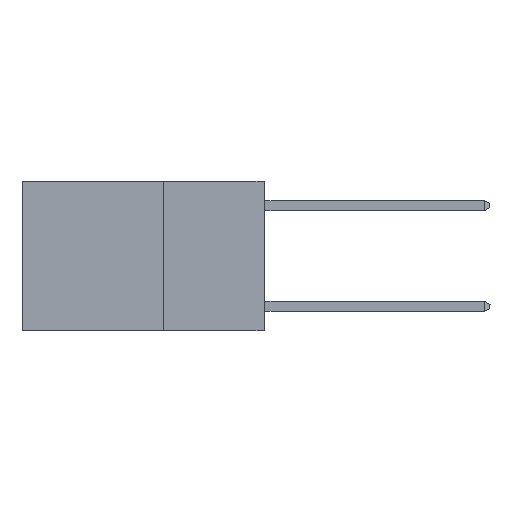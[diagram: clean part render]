
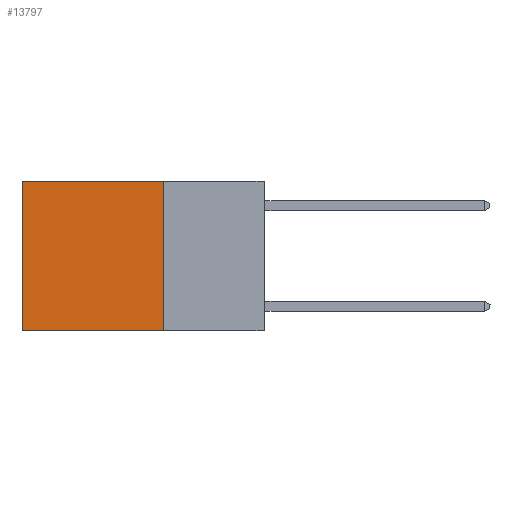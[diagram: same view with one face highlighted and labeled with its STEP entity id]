
A CAD part, left-side view. The second image highlights one B-rep face of the part: STEP entity #13797.
In plain terms, the highlighted planar face has unit normal (-1, 0, 0).
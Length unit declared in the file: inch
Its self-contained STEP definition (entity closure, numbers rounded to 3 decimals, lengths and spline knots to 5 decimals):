
#148 = CARTESIAN_POINT ( 'NONE',  ( 0.2625, 0.25, 0. ) ) ;
#158 = AXIS2_PLACEMENT_3D ( 'NONE', #20457, #4728, #18549 ) ;
#2574 = ORIENTED_EDGE ( 'NONE', *, *, #3627, .T. ) ;
#2757 = PLANE ( 'NONE',  #158 ) ;
#3167 = LINE ( 'NONE', #21795, #13043 ) ;
#3627 = EDGE_CURVE ( 'NONE', #9972, #22703, #16249, .T. ) ;
#4336 = VERTEX_POINT ( 'NONE', #22454 ) ;
#4482 = DIRECTION ( 'NONE',  ( 0., 1., 0. ) ) ;
#4728 = DIRECTION ( 'NONE',  ( 1., 0., 0. ) ) ;
#6208 = EDGE_CURVE ( 'NONE', #4336, #9972, #15558, .T. ) ;
#6687 = DIRECTION ( 'NONE',  ( 0., 0., -1. ) ) ;
#6780 = CARTESIAN_POINT ( 'NONE',  ( 0.2625, 0.6, 0. ) ) ;
#7903 = FACE_OUTER_BOUND ( 'NONE', #21401, .T. ) ;
#8451 = CARTESIAN_POINT ( 'NONE',  ( 0.2625, 0.25, 0. ) ) ;
#8717 = CARTESIAN_POINT ( 'NONE',  ( 0.2625, 0.6, 0. ) ) ;
#9972 = VERTEX_POINT ( 'NONE', #8717 ) ;
#10179 = EDGE_CURVE ( 'NONE', #4336, #18437, #20729, .T. ) ;
#12616 = CARTESIAN_POINT ( 'NONE',  ( 0.2625, 0.6, -0.37 ) ) ;
#13043 = VECTOR ( 'NONE', #17857, 39.37008 ) ;
#13797 = ADVANCED_FACE ( 'NONE', ( #7903 ), #2757, .F. ) ;
#15558 = LINE ( 'NONE', #8451, #20790 ) ;
#16169 = EDGE_CURVE ( 'NONE', #18437, #22703, #3167, .T. ) ;
#16249 = LINE ( 'NONE', #6780, #17508 ) ;
#17508 = VECTOR ( 'NONE', #6687, 39.37008 ) ;
#17857 = DIRECTION ( 'NONE',  ( 0., 1., 0. ) ) ;
#17922 = DIRECTION ( 'NONE',  ( 0., 0., -1. ) ) ;
#18437 = VERTEX_POINT ( 'NONE', #24619 ) ;
#18549 = DIRECTION ( 'NONE',  ( 0., 0., -1. ) ) ;
#20413 = ORIENTED_EDGE ( 'NONE', *, *, #10179, .F. ) ;
#20457 = CARTESIAN_POINT ( 'NONE',  ( 0.2625, 0.25, 0. ) ) ;
#20729 = LINE ( 'NONE', #148, #24608 ) ;
#20790 = VECTOR ( 'NONE', #4482, 39.37008 ) ;
#20835 = ORIENTED_EDGE ( 'NONE', *, *, #16169, .F. ) ;
#21401 = EDGE_LOOP ( 'NONE', ( #2574, #20835, #20413, #24044 ) ) ;
#21795 = CARTESIAN_POINT ( 'NONE',  ( 0.2625, 0.25, -0.37 ) ) ;
#22454 = CARTESIAN_POINT ( 'NONE',  ( 0.2625, 0.25, 0. ) ) ;
#22703 = VERTEX_POINT ( 'NONE', #12616 ) ;
#24044 = ORIENTED_EDGE ( 'NONE', *, *, #6208, .T. ) ;
#24608 = VECTOR ( 'NONE', #17922, 39.37008 ) ;
#24619 = CARTESIAN_POINT ( 'NONE',  ( 0.2625, 0.25, -0.37 ) ) ;
